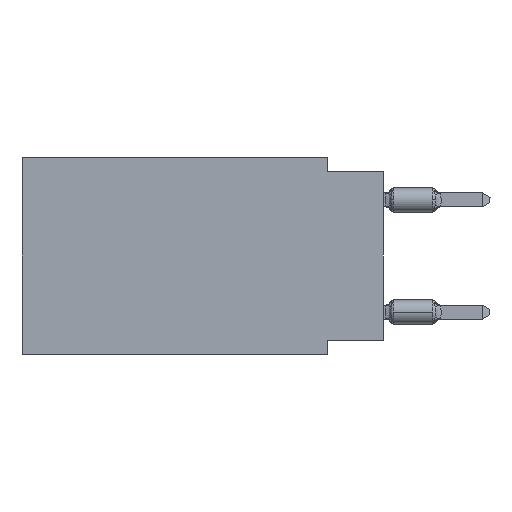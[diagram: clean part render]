
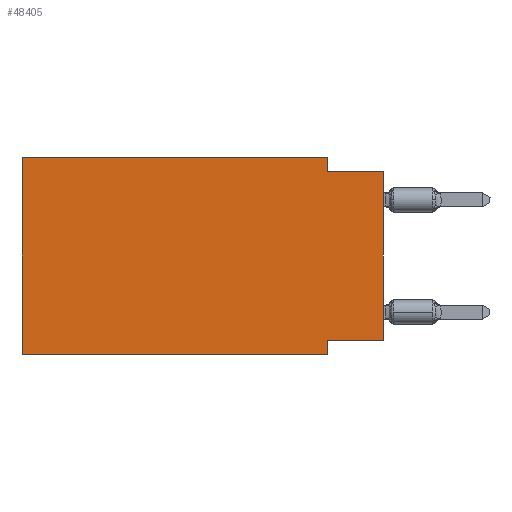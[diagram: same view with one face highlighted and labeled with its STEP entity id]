
A CAD part, left-side view. The second image highlights one B-rep face of the part: STEP entity #48405.
In plain terms, the highlighted planar face has unit normal (-1, 0, 0).
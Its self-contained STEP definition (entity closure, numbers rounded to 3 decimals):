
#315 = VECTOR ( 'NONE', #18700, 1000. ) ;
#533 = FACE_OUTER_BOUND ( 'NONE', #52913, .T. ) ;
#566 = DIRECTION ( 'NONE',  ( 0., 0., -1. ) ) ;
#2005 = VERTEX_POINT ( 'NONE', #57512 ) ;
#3115 = EDGE_CURVE ( 'NONE', #7794, #45895, #36217, .T. ) ;
#3172 = VECTOR ( 'NONE', #33998, 1000. ) ;
#3425 = VECTOR ( 'NONE', #61340, 1000. ) ;
#4686 = CARTESIAN_POINT ( 'NONE',  ( 0., 0., 0. ) ) ;
#7086 = VECTOR ( 'NONE', #26670, 1000. ) ;
#7757 = LINE ( 'NONE', #22382, #25774 ) ;
#7794 = VERTEX_POINT ( 'NONE', #37280 ) ;
#8350 = EDGE_CURVE ( 'NONE', #61000, #51869, #42919, .T. ) ;
#8527 = CARTESIAN_POINT ( 'NONE',  ( 0., 16.383, 0. ) ) ;
#8563 = EDGE_CURVE ( 'NONE', #61000, #12843, #7757, .T. ) ;
#10937 = VERTEX_POINT ( 'NONE', #34631 ) ;
#11666 = CARTESIAN_POINT ( 'NONE',  ( 0., 16.383, 0. ) ) ;
#12026 = ORIENTED_EDGE ( 'NONE', *, *, #8563, .T. ) ;
#12843 = VERTEX_POINT ( 'NONE', #18930 ) ;
#13213 = DIRECTION ( 'NONE',  ( 0., 0., -1. ) ) ;
#14586 = AXIS2_PLACEMENT_3D ( 'NONE', #11666, #40661, #25998 ) ;
#17296 = VECTOR ( 'NONE', #566, 1000. ) ;
#17414 = CARTESIAN_POINT ( 'NONE',  ( 0., 0., -8.255 ) ) ;
#17518 = CARTESIAN_POINT ( 'NONE',  ( 0., 16.383, 0. ) ) ;
#18229 = DIRECTION ( 'NONE',  ( 0., -1., 0. ) ) ;
#18295 = LINE ( 'NONE', #56855, #30764 ) ;
#18700 = DIRECTION ( 'NONE',  ( 0., 0., 1. ) ) ;
#18930 = CARTESIAN_POINT ( 'NONE',  ( 0., 2.54, -8.89 ) ) ;
#20101 = ORIENTED_EDGE ( 'NONE', *, *, #59501, .F. ) ;
#21405 = EDGE_CURVE ( 'NONE', #7794, #10937, #52452, .T. ) ;
#22382 = CARTESIAN_POINT ( 'NONE',  ( 0., 16.383, -8.89 ) ) ;
#23393 = CARTESIAN_POINT ( 'NONE',  ( 0., 2.54, -8.255 ) ) ;
#25774 = VECTOR ( 'NONE', #18229, 1000. ) ;
#25998 = DIRECTION ( 'NONE',  ( 0., 0., -1. ) ) ;
#26670 = DIRECTION ( 'NONE',  ( 0., 1., 0. ) ) ;
#27408 = DIRECTION ( 'NONE',  ( 0., -1., 0. ) ) ;
#28280 = PLANE ( 'NONE',  #14586 ) ;
#28795 = EDGE_CURVE ( 'NONE', #2005, #10937, #61021, .T. ) ;
#28969 = ORIENTED_EDGE ( 'NONE', *, *, #28795, .F. ) ;
#30764 = VECTOR ( 'NONE', #13213, 1000. ) ;
#32196 = ORIENTED_EDGE ( 'NONE', *, *, #8350, .F. ) ;
#33998 = DIRECTION ( 'NONE',  ( 0., 0., 1. ) ) ;
#34631 = CARTESIAN_POINT ( 'NONE',  ( 0., 0., -0.635 ) ) ;
#36217 = LINE ( 'NONE', #17414, #7086 ) ;
#37280 = CARTESIAN_POINT ( 'NONE',  ( 0., 0., -8.255 ) ) ;
#40365 = CARTESIAN_POINT ( 'NONE',  ( 0., 2.54, -8.89 ) ) ;
#40661 = DIRECTION ( 'NONE',  ( 1., 0., 0. ) ) ;
#42919 = LINE ( 'NONE', #8527, #315 ) ;
#43458 = CARTESIAN_POINT ( 'NONE',  ( 0., 16.383, 0. ) ) ;
#44878 = EDGE_CURVE ( 'NONE', #51869, #58788, #61173, .T. ) ;
#45895 = VERTEX_POINT ( 'NONE', #23393 ) ;
#46248 = ORIENTED_EDGE ( 'NONE', *, *, #47028, .F. ) ;
#46555 = ORIENTED_EDGE ( 'NONE', *, *, #44878, .F. ) ;
#47028 = EDGE_CURVE ( 'NONE', #58788, #2005, #18295, .T. ) ;
#47471 = ORIENTED_EDGE ( 'NONE', *, *, #21405, .T. ) ;
#48405 = ADVANCED_FACE ( 'NONE', ( #533 ), #28280, .F. ) ;
#50619 = CARTESIAN_POINT ( 'NONE',  ( 0., 2.54, 0. ) ) ;
#51869 = VERTEX_POINT ( 'NONE', #43458 ) ;
#52452 = LINE ( 'NONE', #4686, #3172 ) ;
#52913 = EDGE_LOOP ( 'NONE', ( #47471, #28969, #46248, #46555, #32196, #12026, #20101, #59783 ) ) ;
#55124 = VECTOR ( 'NONE', #27408, 1000. ) ;
#56232 = CARTESIAN_POINT ( 'NONE',  ( 0., 0., -0.635 ) ) ;
#56855 = CARTESIAN_POINT ( 'NONE',  ( 0., 2.54, 0. ) ) ;
#57512 = CARTESIAN_POINT ( 'NONE',  ( 0., 2.54, -0.635 ) ) ;
#58788 = VERTEX_POINT ( 'NONE', #50619 ) ;
#59501 = EDGE_CURVE ( 'NONE', #45895, #12843, #59817, .T. ) ;
#59783 = ORIENTED_EDGE ( 'NONE', *, *, #3115, .F. ) ;
#59817 = LINE ( 'NONE', #40365, #17296 ) ;
#60532 = CARTESIAN_POINT ( 'NONE',  ( 0., 16.383, -8.89 ) ) ;
#61000 = VERTEX_POINT ( 'NONE', #60532 ) ;
#61021 = LINE ( 'NONE', #56232, #3425 ) ;
#61173 = LINE ( 'NONE', #17518, #55124 ) ;
#61340 = DIRECTION ( 'NONE',  ( 0., -1., 0. ) ) ;
